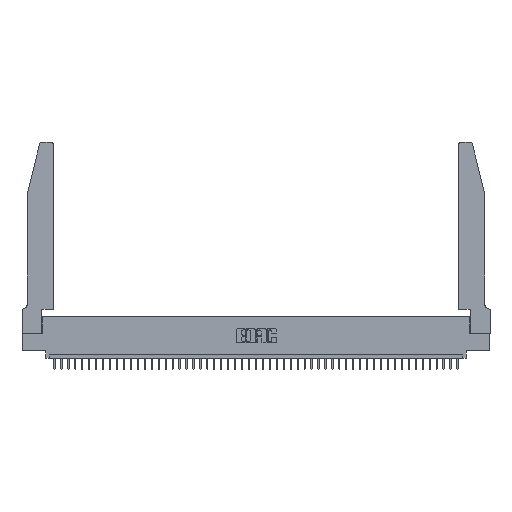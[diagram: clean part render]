
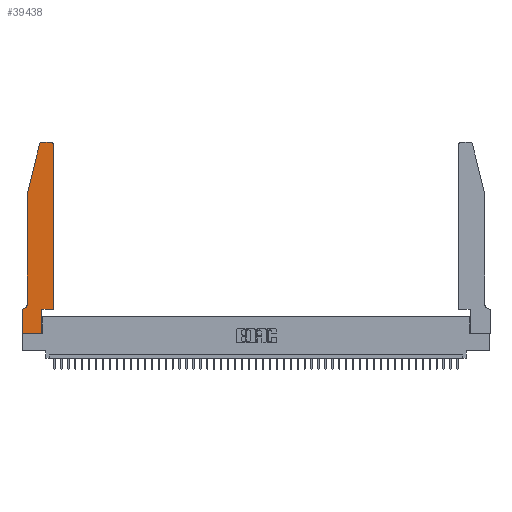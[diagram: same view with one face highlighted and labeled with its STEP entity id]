
A CAD part, top view. The second image highlights one B-rep face of the part: STEP entity #39438.
In plain terms, the highlighted planar face has unit normal (0, 0, 1).
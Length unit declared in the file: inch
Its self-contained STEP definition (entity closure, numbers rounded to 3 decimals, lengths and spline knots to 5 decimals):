
#500 = FACE_OUTER_BOUND ( 'NONE', #34053, .T. ) ;
#630 = ORIENTED_EDGE ( 'NONE', *, *, #34891, .T. ) ;
#1621 = CARTESIAN_POINT ( 'NONE',  ( 0.25487, 2.72718, 0.37 ) ) ;
#1716 = CARTESIAN_POINT ( 'NONE',  ( 0., 0., 0.37 ) ) ;
#1909 = VECTOR ( 'NONE', #24858, 39.37008 ) ;
#3096 = AXIS2_PLACEMENT_3D ( 'NONE', #23625, #28140, #28296 ) ;
#3500 = CARTESIAN_POINT ( 'NONE',  ( 0.4505, 0.35, 0.37 ) ) ;
#4089 = CARTESIAN_POINT ( 'NONE',  ( 0.0755, 2., 0.37 ) ) ;
#7129 = VERTEX_POINT ( 'NONE', #1621 ) ;
#8532 = DIRECTION ( 'NONE',  ( 1., 0., 0. ) ) ;
#8821 = VERTEX_POINT ( 'NONE', #12448 ) ;
#10466 = CIRCLE ( 'NONE', #3096, 0.03 ) ;
#10919 = LINE ( 'NONE', #1716, #24593 ) ;
#10950 = ORIENTED_EDGE ( 'NONE', *, *, #26487, .T. ) ;
#11830 = CARTESIAN_POINT ( 'NONE',  ( 0.4205, 2.72, 0.37 ) ) ;
#12448 = CARTESIAN_POINT ( 'NONE',  ( 0.4205, 2.75, 0.37 ) ) ;
#12636 = AXIS2_PLACEMENT_3D ( 'NONE', #39668, #18015, #8532 ) ;
#12648 = LINE ( 'NONE', #19826, #27417 ) ;
#12751 = DIRECTION ( 'NONE',  ( 1., 0., 0. ) ) ;
#14572 = VECTOR ( 'NONE', #40815, 39.37008 ) ;
#14586 = CIRCLE ( 'NONE', #14943, 0.03 ) ;
#14817 = VECTOR ( 'NONE', #22011, 39.37008 ) ;
#14943 = AXIS2_PLACEMENT_3D ( 'NONE', #11830, #40219, #23287 ) ;
#15001 = ORIENTED_EDGE ( 'NONE', *, *, #33746, .T. ) ;
#15047 = EDGE_CURVE ( 'NONE', #20690, #40950, #45620, .T. ) ;
#15276 = CARTESIAN_POINT ( 'NONE',  ( 0.0755, 2., 0.37 ) ) ;
#16801 = CARTESIAN_POINT ( 'NONE',  ( 0., 0.35, 0.37 ) ) ;
#17362 = CARTESIAN_POINT ( 'NONE',  ( 0.4505, 0.35, 0.37 ) ) ;
#18015 = DIRECTION ( 'NONE',  ( 0., 0., 1. ) ) ;
#18179 = EDGE_CURVE ( 'NONE', #20676, #37542, #36224, .T. ) ;
#18830 = VERTEX_POINT ( 'NONE', #43921 ) ;
#19176 = CARTESIAN_POINT ( 'NONE',  ( 0.0755, 0.35, 0.37 ) ) ;
#19375 = ORIENTED_EDGE ( 'NONE', *, *, #32401, .T. ) ;
#19433 = EDGE_CURVE ( 'NONE', #42887, #24434, #20684, .T. ) ;
#19826 = CARTESIAN_POINT ( 'NONE',  ( 0.2605, 2.75, 0.37 ) ) ;
#20024 = CARTESIAN_POINT ( 'NONE',  ( 0., 0., 0.37 ) ) ;
#20162 = CARTESIAN_POINT ( 'NONE',  ( 0., 0., 0.37 ) ) ;
#20540 = DIRECTION ( 'NONE',  ( 0., -1., 0. ) ) ;
#20635 = EDGE_CURVE ( 'NONE', #40950, #18830, #10919, .T. ) ;
#20676 = VERTEX_POINT ( 'NONE', #42517 ) ;
#20684 = LINE ( 'NONE', #17362, #1909 ) ;
#20690 = VERTEX_POINT ( 'NONE', #16801 ) ;
#20769 = VERTEX_POINT ( 'NONE', #4089 ) ;
#21015 = PLANE ( 'NONE',  #12636 ) ;
#21246 = LINE ( 'NONE', #19176, #37122 ) ;
#22011 = DIRECTION ( 'NONE',  ( 0., -1., 0. ) ) ;
#22940 = VECTOR ( 'NONE', #20540, 39.37008 ) ;
#23084 = LINE ( 'NONE', #15276, #14572 ) ;
#23287 = DIRECTION ( 'NONE',  ( 1., 0., 0. ) ) ;
#23625 = CARTESIAN_POINT ( 'NONE',  ( 0.284, 2.72, 0.37 ) ) ;
#24033 = ORIENTED_EDGE ( 'NONE', *, *, #36136, .T. ) ;
#24285 = AXIS2_PLACEMENT_3D ( 'NONE', #27829, #34958, #27663 ) ;
#24434 = VERTEX_POINT ( 'NONE', #3500 ) ;
#24593 = VECTOR ( 'NONE', #12751, 39.37008 ) ;
#24858 = DIRECTION ( 'NONE',  ( 1., 0., 0. ) ) ;
#24885 = VECTOR ( 'NONE', #29307, 39.37008 ) ;
#25350 = VERTEX_POINT ( 'NONE', #42874 ) ;
#26076 = CARTESIAN_POINT ( 'NONE',  ( 0.284, 2.75, 0.37 ) ) ;
#26452 = ORIENTED_EDGE ( 'NONE', *, *, #46615, .T. ) ;
#26487 = EDGE_CURVE ( 'NONE', #24434, #25350, #41199, .T. ) ;
#27312 = ORIENTED_EDGE ( 'NONE', *, *, #19433, .T. ) ;
#27417 = VECTOR ( 'NONE', #40953, 39.37008 ) ;
#27663 = DIRECTION ( 'NONE',  ( -1., 0., 0. ) ) ;
#27829 = CARTESIAN_POINT ( 'NONE',  ( 0.0055, 0.42, 0.37 ) ) ;
#28140 = DIRECTION ( 'NONE',  ( 0., 0., 1. ) ) ;
#28271 = CARTESIAN_POINT ( 'NONE',  ( 0.0055, 0.35, 0.37 ) ) ;
#28296 = DIRECTION ( 'NONE',  ( 1., 0., 0. ) ) ;
#28421 = EDGE_CURVE ( 'NONE', #8821, #34656, #12648, .T. ) ;
#29061 = CARTESIAN_POINT ( 'NONE',  ( 0.4505, 0.35, 0.37 ) ) ;
#29307 = DIRECTION ( 'NONE',  ( 0., 1., 0. ) ) ;
#29777 = ORIENTED_EDGE ( 'NONE', *, *, #15047, .T. ) ;
#30396 = ORIENTED_EDGE ( 'NONE', *, *, #20635, .T. ) ;
#32401 = EDGE_CURVE ( 'NONE', #18830, #42887, #37367, .T. ) ;
#32733 = EDGE_CURVE ( 'NONE', #7129, #20769, #23084, .T. ) ;
#33746 = EDGE_CURVE ( 'NONE', #20769, #20676, #40654, .T. ) ;
#34053 = EDGE_LOOP ( 'NONE', ( #42399, #630, #40755, #15001, #41807, #26452, #29777, #30396, #19375, #27312, #10950, #24033 ) ) ;
#34656 = VERTEX_POINT ( 'NONE', #26076 ) ;
#34891 = EDGE_CURVE ( 'NONE', #34656, #7129, #10466, .T. ) ;
#34958 = DIRECTION ( 'NONE',  ( 0., 0., -1. ) ) ;
#35322 = CARTESIAN_POINT ( 'NONE',  ( 0.2865, 0.35, 0.37 ) ) ;
#36109 = VECTOR ( 'NONE', #36373, 39.37008 ) ;
#36136 = EDGE_CURVE ( 'NONE', #25350, #8821, #14586, .T. ) ;
#36224 = CIRCLE ( 'NONE', #24285, 0.07 ) ;
#36347 = CARTESIAN_POINT ( 'NONE',  ( 0.2865, 0.35, 0.37 ) ) ;
#36373 = DIRECTION ( 'NONE',  ( 0., 1., 0. ) ) ;
#37122 = VECTOR ( 'NONE', #44682, 39.37008 ) ;
#37367 = LINE ( 'NONE', #36347, #24885 ) ;
#37542 = VERTEX_POINT ( 'NONE', #28271 ) ;
#39438 = ADVANCED_FACE ( 'NONE', ( #500 ), #21015, .T. ) ;
#39668 = CARTESIAN_POINT ( 'NONE',  ( 0., 0.35, 0.37 ) ) ;
#40219 = DIRECTION ( 'NONE',  ( 0., 0., 1. ) ) ;
#40654 = LINE ( 'NONE', #43026, #22940 ) ;
#40755 = ORIENTED_EDGE ( 'NONE', *, *, #32733, .T. ) ;
#40815 = DIRECTION ( 'NONE',  ( -0.239, -0.971, 0. ) ) ;
#40950 = VERTEX_POINT ( 'NONE', #20024 ) ;
#40953 = DIRECTION ( 'NONE',  ( -1., 0., 0. ) ) ;
#41199 = LINE ( 'NONE', #29061, #36109 ) ;
#41807 = ORIENTED_EDGE ( 'NONE', *, *, #18179, .T. ) ;
#42399 = ORIENTED_EDGE ( 'NONE', *, *, #28421, .T. ) ;
#42517 = CARTESIAN_POINT ( 'NONE',  ( 0.0755, 0.42, 0.37 ) ) ;
#42874 = CARTESIAN_POINT ( 'NONE',  ( 0.4505, 2.72, 0.37 ) ) ;
#42887 = VERTEX_POINT ( 'NONE', #35322 ) ;
#43026 = CARTESIAN_POINT ( 'NONE',  ( 0.0755, 2., 0.37 ) ) ;
#43921 = CARTESIAN_POINT ( 'NONE',  ( 0.2865, 0., 0.37 ) ) ;
#44682 = DIRECTION ( 'NONE',  ( -1., 0., 0. ) ) ;
#45620 = LINE ( 'NONE', #20162, #14817 ) ;
#46615 = EDGE_CURVE ( 'NONE', #37542, #20690, #21246, .T. ) ;
